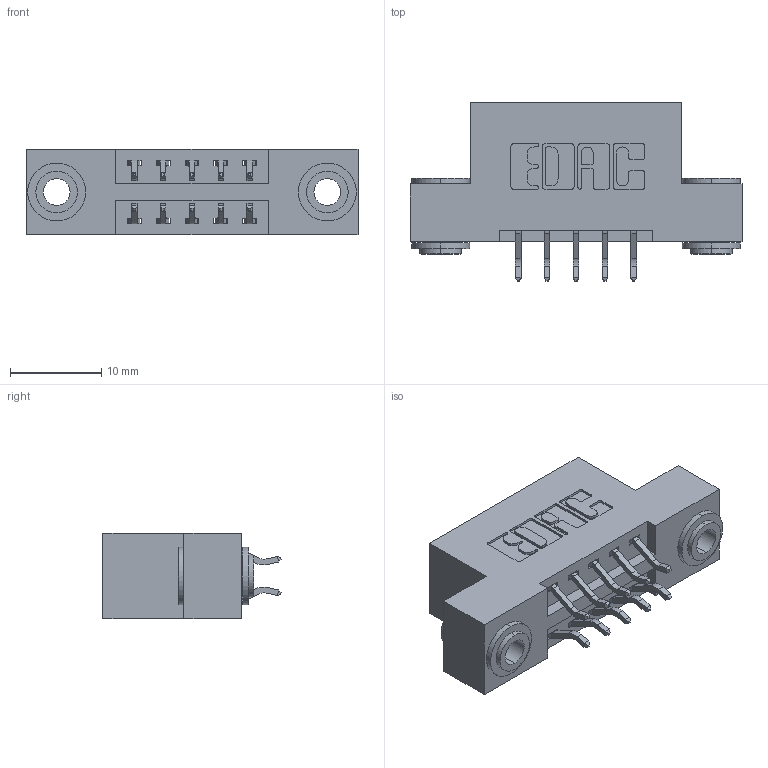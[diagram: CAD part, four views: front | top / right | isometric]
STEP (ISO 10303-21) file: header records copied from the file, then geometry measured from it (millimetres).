
FILE_DESCRIPTION (( 'STEP AP203' ), '1' );
FILE_NAME ('396-010-556-203.STEP', '2018-08-31T03:32:44', ( '' ), ( '' ), 'SwSTEP 2.0', 'SolidWorks 2016', '' );
FILE_SCHEMA (( 'CONFIG_CONTROL_DESIGN' ));
Length unit declared in the file: inch
Products named in the file (4): 346 Part_Flush Mounting Lugs - 0.156 Dia-TH; 345-292-001_556 Tail; 345-250-002_345-250-002-102; 396-010-556-203
Assembly tree (13 placements, depth 2):
  396-010-556-203
    346 Part_Flush Mounting Lugs - 0.156 Dia-TH
    345-292-001_556 Tail  x10
    345-250-002_345-250-002-102  x2
Bounding box: 36.45 x 19.57 x 9.4 mm (x, y, z)
Volume: 3285.9 mm3; surface area: 4140 mm2
Topology: 13 solids, 13 shells, 740 faces, 2135 edges, 1406 vertices
Faces by surface type: plane 476, cylinder 256, cone 8
Entity records: 9114 total; most frequent: CARTESIAN_POINT 1543, ORIENTED_EDGE 1458, DIRECTION 1431, EDGE_CURVE 729, LINE 545, VECTOR 545, VERTEX_POINT 482, AXIS2_PLACEMENT_3D 443
